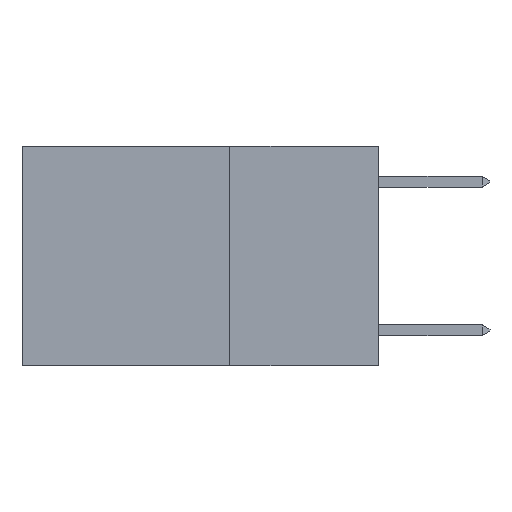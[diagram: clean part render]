
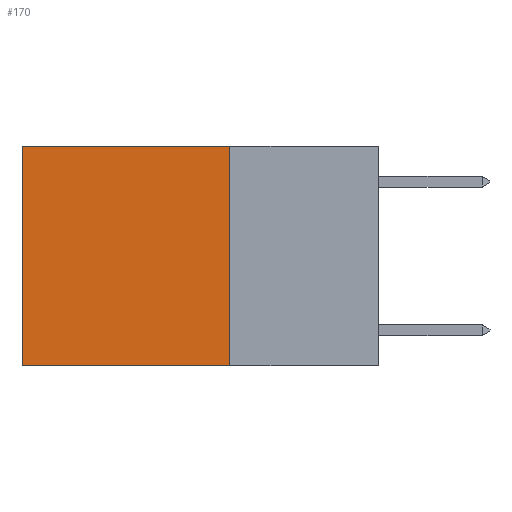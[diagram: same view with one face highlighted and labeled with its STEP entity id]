
A CAD part, left-side view. The second image highlights one B-rep face of the part: STEP entity #170.
In plain terms, the highlighted planar face has unit normal (-1, 0, 0).
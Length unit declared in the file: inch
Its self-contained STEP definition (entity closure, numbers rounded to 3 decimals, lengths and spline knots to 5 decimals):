
#170 = ADVANCED_FACE ( 'NONE', ( #9084 ), #6394, .F. ) ;
#205 = AXIS2_PLACEMENT_3D ( 'NONE', #7514, #8977, #8849 ) ;
#1225 = DIRECTION ( 'NONE',  ( 0., 1., 0. ) ) ;
#1569 = EDGE_CURVE ( 'NONE', #9034, #2137, #5507, .T. ) ;
#1657 = ORIENTED_EDGE ( 'NONE', *, *, #4262, .T. ) ;
#2137 = VERTEX_POINT ( 'NONE', #3212 ) ;
#2465 = CARTESIAN_POINT ( 'NONE',  ( 0.2625, 0.6, 0. ) ) ;
#2588 = ORIENTED_EDGE ( 'NONE', *, *, #9964, .T. ) ;
#3212 = CARTESIAN_POINT ( 'NONE',  ( 0.2625, 0.25, -0.37 ) ) ;
#4081 = ORIENTED_EDGE ( 'NONE', *, *, #5349, .F. ) ;
#4262 = EDGE_CURVE ( 'NONE', #6130, #7034, #9963, .T. ) ;
#4497 = CARTESIAN_POINT ( 'NONE',  ( 0.2625, 0.25, 0. ) ) ;
#4803 = DIRECTION ( 'NONE',  ( 0., 1., 0. ) ) ;
#5349 = EDGE_CURVE ( 'NONE', #2137, #7034, #7333, .T. ) ;
#5444 = CARTESIAN_POINT ( 'NONE',  ( 0.2625, 0.6, 0. ) ) ;
#5507 = LINE ( 'NONE', #9740, #9640 ) ;
#5625 = VECTOR ( 'NONE', #9130, 39.37008 ) ;
#6130 = VERTEX_POINT ( 'NONE', #5444 ) ;
#6239 = ORIENTED_EDGE ( 'NONE', *, *, #1569, .F. ) ;
#6394 = PLANE ( 'NONE',  #205 ) ;
#6995 = VECTOR ( 'NONE', #4803, 39.37008 ) ;
#7034 = VERTEX_POINT ( 'NONE', #7353 ) ;
#7077 = VECTOR ( 'NONE', #1225, 39.37008 ) ;
#7333 = LINE ( 'NONE', #7950, #7077 ) ;
#7353 = CARTESIAN_POINT ( 'NONE',  ( 0.2625, 0.6, -0.37 ) ) ;
#7514 = CARTESIAN_POINT ( 'NONE',  ( 0.2625, 0.25, 0. ) ) ;
#7703 = EDGE_LOOP ( 'NONE', ( #1657, #4081, #6239, #2588 ) ) ;
#7950 = CARTESIAN_POINT ( 'NONE',  ( 0.2625, 0.25, -0.37 ) ) ;
#8220 = DIRECTION ( 'NONE',  ( 0., 0., -1. ) ) ;
#8849 = DIRECTION ( 'NONE',  ( 0., 0., -1. ) ) ;
#8944 = LINE ( 'NONE', #10485, #6995 ) ;
#8977 = DIRECTION ( 'NONE',  ( 1., 0., 0. ) ) ;
#9034 = VERTEX_POINT ( 'NONE', #4497 ) ;
#9084 = FACE_OUTER_BOUND ( 'NONE', #7703, .T. ) ;
#9130 = DIRECTION ( 'NONE',  ( 0., 0., -1. ) ) ;
#9640 = VECTOR ( 'NONE', #8220, 39.37008 ) ;
#9740 = CARTESIAN_POINT ( 'NONE',  ( 0.2625, 0.25, 0. ) ) ;
#9963 = LINE ( 'NONE', #2465, #5625 ) ;
#9964 = EDGE_CURVE ( 'NONE', #9034, #6130, #8944, .T. ) ;
#10485 = CARTESIAN_POINT ( 'NONE',  ( 0.2625, 0.25, 0. ) ) ;
